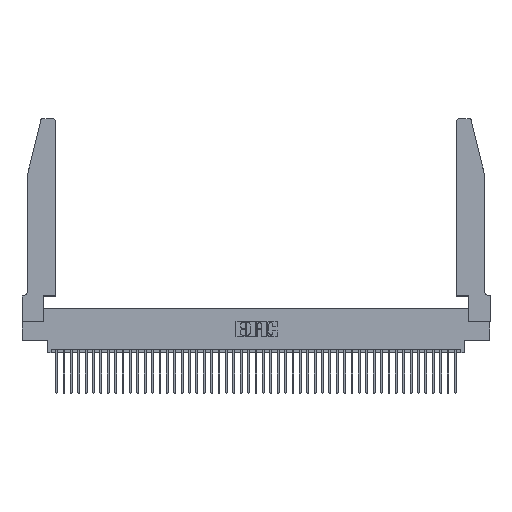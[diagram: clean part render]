
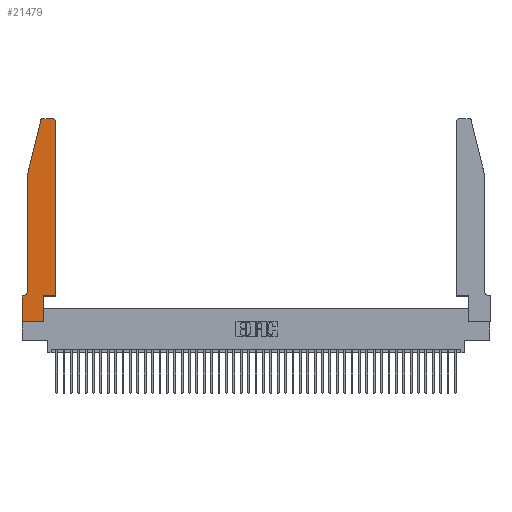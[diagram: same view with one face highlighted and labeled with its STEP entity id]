
A CAD part, top view. The second image highlights one B-rep face of the part: STEP entity #21479.
In plain terms, the highlighted planar face has unit normal (0, 0, 1).
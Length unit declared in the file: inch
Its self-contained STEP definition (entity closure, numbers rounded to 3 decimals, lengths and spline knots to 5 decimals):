
#181 = CARTESIAN_POINT ( 'NONE',  ( 0.0755, 0.42, 0.37 ) ) ;
#383 = ORIENTED_EDGE ( 'NONE', *, *, #46149, .T. ) ;
#1097 = CARTESIAN_POINT ( 'NONE',  ( 0.2865, 0., 0.37 ) ) ;
#1658 = VECTOR ( 'NONE', #17139, 39.37008 ) ;
#1726 = CARTESIAN_POINT ( 'NONE',  ( 0.4505, 2.72, 0.37 ) ) ;
#2250 = ORIENTED_EDGE ( 'NONE', *, *, #39649, .T. ) ;
#3452 = LINE ( 'NONE', #33934, #38691 ) ;
#3565 = VERTEX_POINT ( 'NONE', #6912 ) ;
#3764 = LINE ( 'NONE', #8230, #15551 ) ;
#4050 = CARTESIAN_POINT ( 'NONE',  ( 0., 0., 0.37 ) ) ;
#4564 = ORIENTED_EDGE ( 'NONE', *, *, #19206, .T. ) ;
#4775 = ORIENTED_EDGE ( 'NONE', *, *, #34312, .T. ) ;
#4820 = DIRECTION ( 'NONE',  ( -0.239, -0.971, 0. ) ) ;
#4964 = ORIENTED_EDGE ( 'NONE', *, *, #35687, .T. ) ;
#6302 = VECTOR ( 'NONE', #41219, 39.37008 ) ;
#6323 = VERTEX_POINT ( 'NONE', #4050 ) ;
#6559 = VERTEX_POINT ( 'NONE', #1726 ) ;
#6639 = LINE ( 'NONE', #35615, #23424 ) ;
#6649 = FACE_OUTER_BOUND ( 'NONE', #43030, .T. ) ;
#6912 = CARTESIAN_POINT ( 'NONE',  ( 0.25487, 2.72718, 0.37 ) ) ;
#7908 = DIRECTION ( 'NONE',  ( 0., -1., 0. ) ) ;
#8230 = CARTESIAN_POINT ( 'NONE',  ( 0.0755, 2., 0.37 ) ) ;
#8537 = CARTESIAN_POINT ( 'NONE',  ( 0., 0.35, 0.37 ) ) ;
#8696 = AXIS2_PLACEMENT_3D ( 'NONE', #36235, #40084, #21971 ) ;
#8891 = CIRCLE ( 'NONE', #9252, 0.07 ) ;
#8928 = LINE ( 'NONE', #31364, #1658 ) ;
#9252 = AXIS2_PLACEMENT_3D ( 'NONE', #10547, #14290, #24858 ) ;
#9578 = CARTESIAN_POINT ( 'NONE',  ( 0., 0., 0.37 ) ) ;
#10324 = CARTESIAN_POINT ( 'NONE',  ( 0.0755, 0.35, 0.37 ) ) ;
#10547 = CARTESIAN_POINT ( 'NONE',  ( 0.0055, 0.42, 0.37 ) ) ;
#11202 = PLANE ( 'NONE',  #8696 ) ;
#11668 = CARTESIAN_POINT ( 'NONE',  ( 0.2865, 0.35, 0.37 ) ) ;
#11892 = VERTEX_POINT ( 'NONE', #12900 ) ;
#12068 = LINE ( 'NONE', #9578, #26607 ) ;
#12580 = CARTESIAN_POINT ( 'NONE',  ( 0.2605, 2.75, 0.37 ) ) ;
#12835 = VECTOR ( 'NONE', #16646, 39.37008 ) ;
#12900 = CARTESIAN_POINT ( 'NONE',  ( 0.0755, 2., 0.37 ) ) ;
#13344 = ORIENTED_EDGE ( 'NONE', *, *, #32635, .T. ) ;
#13552 = DIRECTION ( 'NONE',  ( 0., 0., 1. ) ) ;
#13579 = ORIENTED_EDGE ( 'NONE', *, *, #33619, .T. ) ;
#13653 = VECTOR ( 'NONE', #32380, 39.37008 ) ;
#14035 = DIRECTION ( 'NONE',  ( 1., 0., 0. ) ) ;
#14290 = DIRECTION ( 'NONE',  ( 0., 0., -1. ) ) ;
#14872 = CARTESIAN_POINT ( 'NONE',  ( 0.4205, 2.75, 0.37 ) ) ;
#15551 = VECTOR ( 'NONE', #7908, 39.37008 ) ;
#15997 = VERTEX_POINT ( 'NONE', #11668 ) ;
#16646 = DIRECTION ( 'NONE',  ( -1., 0., 0. ) ) ;
#16838 = CARTESIAN_POINT ( 'NONE',  ( 0.0055, 0.35, 0.37 ) ) ;
#17139 = DIRECTION ( 'NONE',  ( 0., 1., 0. ) ) ;
#19206 = EDGE_CURVE ( 'NONE', #32236, #15997, #39828, .T. ) ;
#21019 = CARTESIAN_POINT ( 'NONE',  ( 0.284, 2.72, 0.37 ) ) ;
#21479 = ADVANCED_FACE ( 'NONE', ( #6649 ), #11202, .T. ) ;
#21598 = VERTEX_POINT ( 'NONE', #16838 ) ;
#21971 = DIRECTION ( 'NONE',  ( 1., 0., 0. ) ) ;
#23424 = VECTOR ( 'NONE', #14035, 39.37008 ) ;
#24590 = VERTEX_POINT ( 'NONE', #8537 ) ;
#24858 = DIRECTION ( 'NONE',  ( -1., 0., 0. ) ) ;
#25782 = VERTEX_POINT ( 'NONE', #37220 ) ;
#25897 = CARTESIAN_POINT ( 'NONE',  ( 0.2865, 0.35, 0.37 ) ) ;
#26368 = VERTEX_POINT ( 'NONE', #45374 ) ;
#26607 = VECTOR ( 'NONE', #41915, 39.37008 ) ;
#26882 = ORIENTED_EDGE ( 'NONE', *, *, #26891, .T. ) ;
#26891 = EDGE_CURVE ( 'NONE', #15997, #26368, #34318, .T. ) ;
#28324 = CARTESIAN_POINT ( 'NONE',  ( 0.4505, 0.35, 0.37 ) ) ;
#29769 = LINE ( 'NONE', #10324, #39745 ) ;
#31096 = ORIENTED_EDGE ( 'NONE', *, *, #37461, .T. ) ;
#31364 = CARTESIAN_POINT ( 'NONE',  ( 0.4505, 0.35, 0.37 ) ) ;
#32129 = VERTEX_POINT ( 'NONE', #14872 ) ;
#32236 = VERTEX_POINT ( 'NONE', #1097 ) ;
#32363 = AXIS2_PLACEMENT_3D ( 'NONE', #21019, #13552, #42274 ) ;
#32380 = DIRECTION ( 'NONE',  ( 1., 0., 0. ) ) ;
#32635 = EDGE_CURVE ( 'NONE', #6323, #32236, #6639, .T. ) ;
#33619 = EDGE_CURVE ( 'NONE', #6559, #32129, #44951, .T. ) ;
#33934 = CARTESIAN_POINT ( 'NONE',  ( 0.0755, 2., 0.37 ) ) ;
#34177 = AXIS2_PLACEMENT_3D ( 'NONE', #36181, #43976, #36334 ) ;
#34312 = EDGE_CURVE ( 'NONE', #3565, #11892, #3452, .T. ) ;
#34318 = LINE ( 'NONE', #28324, #13653 ) ;
#35237 = LINE ( 'NONE', #12580, #12835 ) ;
#35314 = DIRECTION ( 'NONE',  ( -1., 0., 0. ) ) ;
#35615 = CARTESIAN_POINT ( 'NONE',  ( 0., 0., 0.37 ) ) ;
#35621 = ORIENTED_EDGE ( 'NONE', *, *, #43650, .T. ) ;
#35687 = EDGE_CURVE ( 'NONE', #26368, #6559, #8928, .T. ) ;
#35879 = ORIENTED_EDGE ( 'NONE', *, *, #38463, .T. ) ;
#35923 = VERTEX_POINT ( 'NONE', #181 ) ;
#36181 = CARTESIAN_POINT ( 'NONE',  ( 0.4205, 2.72, 0.37 ) ) ;
#36235 = CARTESIAN_POINT ( 'NONE',  ( 0., 0.35, 0.37 ) ) ;
#36334 = DIRECTION ( 'NONE',  ( 1., 0., 0. ) ) ;
#37220 = CARTESIAN_POINT ( 'NONE',  ( 0.284, 2.75, 0.37 ) ) ;
#37461 = EDGE_CURVE ( 'NONE', #11892, #35923, #3764, .T. ) ;
#38463 = EDGE_CURVE ( 'NONE', #25782, #3565, #42828, .T. ) ;
#38678 = ORIENTED_EDGE ( 'NONE', *, *, #46022, .T. ) ;
#38691 = VECTOR ( 'NONE', #4820, 39.37008 ) ;
#39649 = EDGE_CURVE ( 'NONE', #21598, #24590, #29769, .T. ) ;
#39745 = VECTOR ( 'NONE', #35314, 39.37008 ) ;
#39828 = LINE ( 'NONE', #25897, #6302 ) ;
#40084 = DIRECTION ( 'NONE',  ( 0., 0., 1. ) ) ;
#41219 = DIRECTION ( 'NONE',  ( 0., 1., 0. ) ) ;
#41915 = DIRECTION ( 'NONE',  ( 0., -1., 0. ) ) ;
#42274 = DIRECTION ( 'NONE',  ( 1., 0., 0. ) ) ;
#42828 = CIRCLE ( 'NONE', #32363, 0.03 ) ;
#43030 = EDGE_LOOP ( 'NONE', ( #38678, #35879, #4775, #31096, #383, #2250, #35621, #13344, #4564, #26882, #4964, #13579 ) ) ;
#43650 = EDGE_CURVE ( 'NONE', #24590, #6323, #12068, .T. ) ;
#43976 = DIRECTION ( 'NONE',  ( 0., 0., 1. ) ) ;
#44951 = CIRCLE ( 'NONE', #34177, 0.03 ) ;
#45374 = CARTESIAN_POINT ( 'NONE',  ( 0.4505, 0.35, 0.37 ) ) ;
#46022 = EDGE_CURVE ( 'NONE', #32129, #25782, #35237, .T. ) ;
#46149 = EDGE_CURVE ( 'NONE', #35923, #21598, #8891, .T. ) ;
